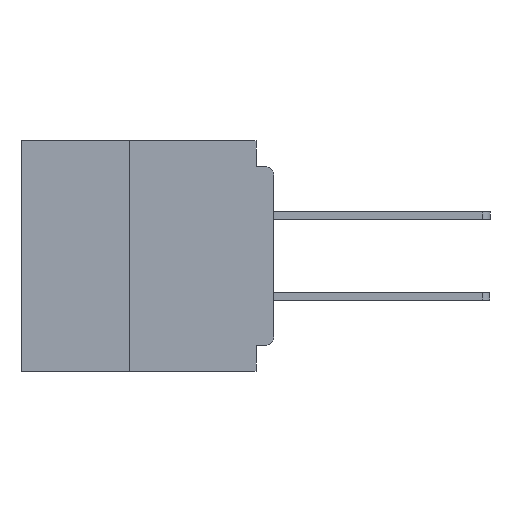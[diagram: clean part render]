
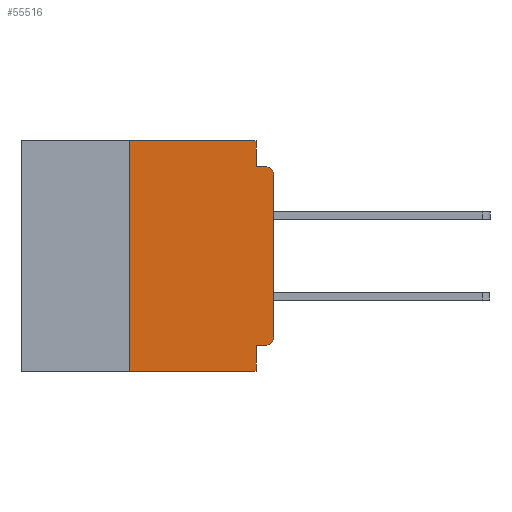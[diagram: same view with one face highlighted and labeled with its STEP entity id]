
A CAD part, left-side view. The second image highlights one B-rep face of the part: STEP entity #55516.
In plain terms, the highlighted planar face has unit normal (-1, 0, 0).
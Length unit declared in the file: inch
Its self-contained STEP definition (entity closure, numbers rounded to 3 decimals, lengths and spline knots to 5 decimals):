
#32 = LINE ( 'NONE', #11048, #21680 ) ;
#34 = VERTEX_POINT ( 'NONE', #9346 ) ;
#1886 = EDGE_CURVE ( 'NONE', #55068, #9652, #51144, .T. ) ;
#4387 = LINE ( 'NONE', #20607, #17248 ) ;
#4613 = DIRECTION ( 'NONE',  ( 0., 0., -1. ) ) ;
#4870 = VERTEX_POINT ( 'NONE', #20854 ) ;
#5486 = CARTESIAN_POINT ( 'NONE',  ( 0., 0.015, -0.355 ) ) ;
#5587 = VECTOR ( 'NONE', #12536, 39.37008 ) ;
#6092 = CARTESIAN_POINT ( 'NONE',  ( 0., 0.031, -0.045 ) ) ;
#6178 = CIRCLE ( 'NONE', #44423, 0.015 ) ;
#6488 = VERTEX_POINT ( 'NONE', #24382 ) ;
#9022 = CARTESIAN_POINT ( 'NONE',  ( 0., 0.031, -0.4 ) ) ;
#9078 = VECTOR ( 'NONE', #4613, 39.37008 ) ;
#9346 = CARTESIAN_POINT ( 'NONE',  ( 0., 0.031, 0. ) ) ;
#9520 = ORIENTED_EDGE ( 'NONE', *, *, #20920, .T. ) ;
#9652 = VERTEX_POINT ( 'NONE', #14860 ) ;
#10686 = AXIS2_PLACEMENT_3D ( 'NONE', #49895, #24325, #54187 ) ;
#11048 = CARTESIAN_POINT ( 'NONE',  ( 0., 0.031, 0. ) ) ;
#12454 = CARTESIAN_POINT ( 'NONE',  ( 0., 0., -0.045 ) ) ;
#12536 = DIRECTION ( 'NONE',  ( 0., -1., 0. ) ) ;
#12630 = VECTOR ( 'NONE', #44293, 39.37008 ) ;
#12681 = CARTESIAN_POINT ( 'NONE',  ( 0., 0.437, 0. ) ) ;
#13070 = VERTEX_POINT ( 'NONE', #5486 ) ;
#13125 = ORIENTED_EDGE ( 'NONE', *, *, #54481, .T. ) ;
#14012 = CARTESIAN_POINT ( 'NONE',  ( 0., 0.437, 0. ) ) ;
#14107 = VERTEX_POINT ( 'NONE', #41309 ) ;
#14419 = CARTESIAN_POINT ( 'NONE',  ( 0., 0., 0. ) ) ;
#14860 = CARTESIAN_POINT ( 'NONE',  ( 0., 0.015, -0.045 ) ) ;
#15377 = DIRECTION ( 'NONE',  ( 0., 0., -1. ) ) ;
#15416 = DIRECTION ( 'NONE',  ( -1., 0., 0. ) ) ;
#15987 = EDGE_CURVE ( 'NONE', #13070, #37509, #4387, .T. ) ;
#17248 = VECTOR ( 'NONE', #24863, 39.37008 ) ;
#17900 = ORIENTED_EDGE ( 'NONE', *, *, #52847, .F. ) ;
#19292 = LINE ( 'NONE', #19430, #52051 ) ;
#19430 = CARTESIAN_POINT ( 'NONE',  ( 0., 0.25, -0.4 ) ) ;
#20607 = CARTESIAN_POINT ( 'NONE',  ( 0., 0., -0.355 ) ) ;
#20854 = CARTESIAN_POINT ( 'NONE',  ( 0., 0.031, -0.4 ) ) ;
#20920 = EDGE_CURVE ( 'NONE', #6488, #4870, #33298, .T. ) ;
#21680 = VECTOR ( 'NONE', #15377, 39.37008 ) ;
#22293 = EDGE_CURVE ( 'NONE', #37509, #4870, #33141, .T. ) ;
#22799 = DIRECTION ( 'NONE',  ( 0., 0., -1. ) ) ;
#24325 = DIRECTION ( 'NONE',  ( -1., 0., 0. ) ) ;
#24382 = CARTESIAN_POINT ( 'NONE',  ( 0., 0.25, -0.4 ) ) ;
#24863 = DIRECTION ( 'NONE',  ( 0., 1., 0. ) ) ;
#26134 = EDGE_CURVE ( 'NONE', #13070, #26548, #42221, .T. ) ;
#26467 = DIRECTION ( 'NONE',  ( 0., -1., 0. ) ) ;
#26548 = VERTEX_POINT ( 'NONE', #52649 ) ;
#27435 = ORIENTED_EDGE ( 'NONE', *, *, #52609, .F. ) ;
#32651 = EDGE_CURVE ( 'NONE', #26548, #50160, #35336, .T. ) ;
#33000 = ORIENTED_EDGE ( 'NONE', *, *, #1886, .F. ) ;
#33141 = LINE ( 'NONE', #9022, #9078 ) ;
#33298 = LINE ( 'NONE', #47931, #53337 ) ;
#34422 = AXIS2_PLACEMENT_3D ( 'NONE', #14012, #48359, #22799 ) ;
#34880 = FACE_OUTER_BOUND ( 'NONE', #47464, .T. ) ;
#35336 = LINE ( 'NONE', #14419, #12630 ) ;
#37509 = VERTEX_POINT ( 'NONE', #54524 ) ;
#37898 = CARTESIAN_POINT ( 'NONE',  ( 0., 0., -0.06 ) ) ;
#38356 = ORIENTED_EDGE ( 'NONE', *, *, #22293, .F. ) ;
#39960 = VECTOR ( 'NONE', #55434, 39.37008 ) ;
#40117 = ORIENTED_EDGE ( 'NONE', *, *, #32651, .T. ) ;
#40980 = CARTESIAN_POINT ( 'NONE',  ( 0., 0.015, -0.06 ) ) ;
#41309 = CARTESIAN_POINT ( 'NONE',  ( 0., 0.25, 0. ) ) ;
#42221 = CIRCLE ( 'NONE', #10686, 0.015 ) ;
#42789 = ORIENTED_EDGE ( 'NONE', *, *, #46091, .F. ) ;
#44070 = PLANE ( 'NONE',  #34422 ) ;
#44293 = DIRECTION ( 'NONE',  ( 0., 0., 1. ) ) ;
#44423 = AXIS2_PLACEMENT_3D ( 'NONE', #40980, #15416, #45290 ) ;
#45290 = DIRECTION ( 'NONE',  ( 0., 0., -1. ) ) ;
#46091 = EDGE_CURVE ( 'NONE', #34, #55068, #32, .T. ) ;
#47464 = EDGE_LOOP ( 'NONE', ( #40117, #13125, #33000, #42789, #17900, #27435, #9520, #38356, #52878, #54321 ) ) ;
#47931 = CARTESIAN_POINT ( 'NONE',  ( 0., 0.437, -0.4 ) ) ;
#48359 = DIRECTION ( 'NONE',  ( 1., 0., 0. ) ) ;
#49312 = DIRECTION ( 'NONE',  ( 0., 0., 1. ) ) ;
#49895 = CARTESIAN_POINT ( 'NONE',  ( 0., 0.015, -0.34 ) ) ;
#50160 = VERTEX_POINT ( 'NONE', #37898 ) ;
#51144 = LINE ( 'NONE', #12454, #5587 ) ;
#51369 = LINE ( 'NONE', #12681, #39960 ) ;
#52051 = VECTOR ( 'NONE', #49312, 39.37008 ) ;
#52609 = EDGE_CURVE ( 'NONE', #6488, #14107, #19292, .T. ) ;
#52649 = CARTESIAN_POINT ( 'NONE',  ( 0., 0., -0.34 ) ) ;
#52847 = EDGE_CURVE ( 'NONE', #14107, #34, #51369, .T. ) ;
#52878 = ORIENTED_EDGE ( 'NONE', *, *, #15987, .F. ) ;
#53337 = VECTOR ( 'NONE', #26467, 39.37008 ) ;
#54187 = DIRECTION ( 'NONE',  ( 0., 0., -1. ) ) ;
#54321 = ORIENTED_EDGE ( 'NONE', *, *, #26134, .T. ) ;
#54481 = EDGE_CURVE ( 'NONE', #50160, #9652, #6178, .T. ) ;
#54524 = CARTESIAN_POINT ( 'NONE',  ( 0., 0.031, -0.355 ) ) ;
#55068 = VERTEX_POINT ( 'NONE', #6092 ) ;
#55434 = DIRECTION ( 'NONE',  ( 0., -1., 0. ) ) ;
#55516 = ADVANCED_FACE ( 'NONE', ( #34880 ), #44070, .F. ) ;
